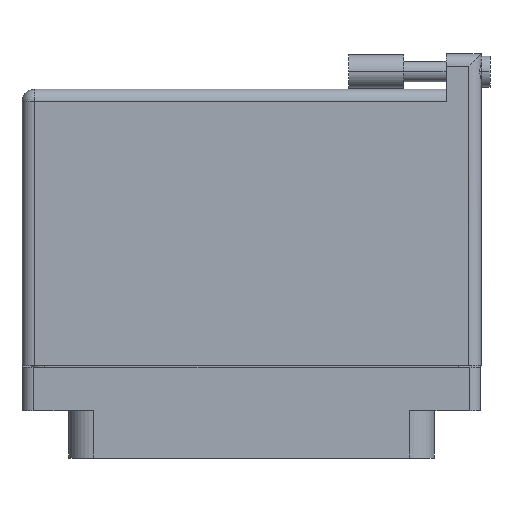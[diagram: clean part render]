
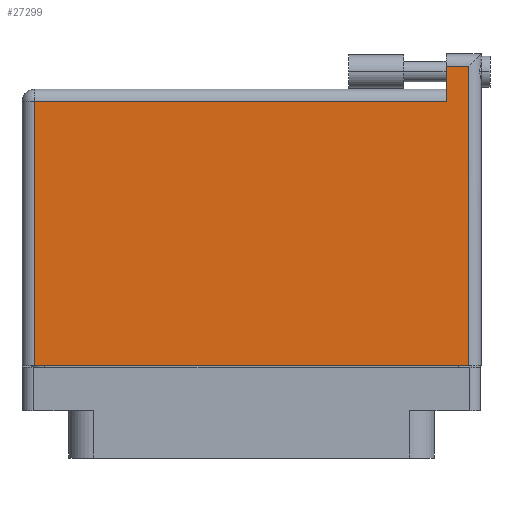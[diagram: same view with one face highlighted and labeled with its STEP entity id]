
A CAD part, front view. The second image highlights one B-rep face of the part: STEP entity #27299.
In plain terms, the highlighted face is planar.
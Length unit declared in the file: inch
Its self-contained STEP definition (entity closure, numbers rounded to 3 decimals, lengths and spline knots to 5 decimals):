
#318 = EDGE_LOOP ( 'NONE', ( #650, #1971, #25105, #33559, #22219, #26709 ) ) ;
#485 = DIRECTION ( 'NONE',  ( -1., 0., 0. ) ) ;
#650 = ORIENTED_EDGE ( 'NONE', *, *, #10344, .T. ) ;
#1971 = ORIENTED_EDGE ( 'NONE', *, *, #14185, .T. ) ;
#2944 = CARTESIAN_POINT ( 'NONE',  ( 1.23, 1.596, 0.4495 ) ) ;
#4171 = LINE ( 'NONE', #36304, #36687 ) ;
#6224 = CARTESIAN_POINT ( 'NONE',  ( -1.3, 1.396, 0.4495 ) ) ;
#7894 = CARTESIAN_POINT ( 'NONE',  ( -1.23, -0.1, 0.4495 ) ) ;
#9445 = VECTOR ( 'NONE', #18365, 39.37008 ) ;
#9795 = CARTESIAN_POINT ( 'NONE',  ( -1.3, 1.466, 0.4495 ) ) ;
#10344 = EDGE_CURVE ( 'NONE', #38540, #32235, #38788, .T. ) ;
#11542 = DIRECTION ( 'NONE',  ( 0., -1., 0. ) ) ;
#11992 = VECTOR ( 'NONE', #11542, 39.37008 ) ;
#13649 = LINE ( 'NONE', #29604, #9445 ) ;
#14185 = EDGE_CURVE ( 'NONE', #32235, #29164, #13649, .T. ) ;
#18365 = DIRECTION ( 'NONE',  ( 0., 1., 0. ) ) ;
#19514 = VERTEX_POINT ( 'NONE', #51599 ) ;
#22219 = ORIENTED_EDGE ( 'NONE', *, *, #42935, .T. ) ;
#25105 = ORIENTED_EDGE ( 'NONE', *, *, #32129, .T. ) ;
#25746 = PLANE ( 'NONE',  #43138 ) ;
#26006 = FACE_OUTER_BOUND ( 'NONE', #318, .T. ) ;
#26104 = LINE ( 'NONE', #6224, #44532 ) ;
#26105 = CARTESIAN_POINT ( 'NONE',  ( 1.23, -0.1, 0.4495 ) ) ;
#26254 = VECTOR ( 'NONE', #30962, 39.37008 ) ;
#26709 = ORIENTED_EDGE ( 'NONE', *, *, #37943, .T. ) ;
#27299 = ADVANCED_FACE ( 'NONE', ( #26006 ), #25746, .F. ) ;
#29164 = VERTEX_POINT ( 'NONE', #2944 ) ;
#29511 = DIRECTION ( 'NONE',  ( -1., 0., 0. ) ) ;
#29604 = CARTESIAN_POINT ( 'NONE',  ( 1.23, 1.666, 0.4495 ) ) ;
#30738 = CARTESIAN_POINT ( 'NONE',  ( 1.103, 1.666, 0.4495 ) ) ;
#30962 = DIRECTION ( 'NONE',  ( 1., 0., 0. ) ) ;
#32129 = EDGE_CURVE ( 'NONE', #29164, #34216, #4171, .T. ) ;
#32235 = VERTEX_POINT ( 'NONE', #26105 ) ;
#32478 = LINE ( 'NONE', #7894, #11992 ) ;
#32806 = EDGE_CURVE ( 'NONE', #34216, #33630, #34902, .T. ) ;
#32936 = CARTESIAN_POINT ( 'NONE',  ( -1.23, -0.1, 0.4495 ) ) ;
#33559 = ORIENTED_EDGE ( 'NONE', *, *, #32806, .T. ) ;
#33630 = VERTEX_POINT ( 'NONE', #35743 ) ;
#34216 = VERTEX_POINT ( 'NONE', #34673 ) ;
#34409 = DIRECTION ( 'NONE',  ( 0., -1., 0. ) ) ;
#34673 = CARTESIAN_POINT ( 'NONE',  ( 1.103, 1.596, 0.4495 ) ) ;
#34902 = LINE ( 'NONE', #30738, #40949 ) ;
#35743 = CARTESIAN_POINT ( 'NONE',  ( 1.103, 1.396, 0.4495 ) ) ;
#36304 = CARTESIAN_POINT ( 'NONE',  ( -1.3, 1.596, 0.4495 ) ) ;
#36687 = VECTOR ( 'NONE', #485, 39.37008 ) ;
#37943 = EDGE_CURVE ( 'NONE', #19514, #38540, #32478, .T. ) ;
#38540 = VERTEX_POINT ( 'NONE', #32936 ) ;
#38788 = LINE ( 'NONE', #39036, #26254 ) ;
#39036 = CARTESIAN_POINT ( 'NONE',  ( -1.3, -0.1, 0.4495 ) ) ;
#40949 = VECTOR ( 'NONE', #34409, 39.37008 ) ;
#41683 = DIRECTION ( 'NONE',  ( -1., 0., 0. ) ) ;
#42935 = EDGE_CURVE ( 'NONE', #33630, #19514, #26104, .T. ) ;
#43138 = AXIS2_PLACEMENT_3D ( 'NONE', #9795, #45093, #41683 ) ;
#44532 = VECTOR ( 'NONE', #29511, 39.37008 ) ;
#45093 = DIRECTION ( 'NONE',  ( 0., 0., -1. ) ) ;
#51599 = CARTESIAN_POINT ( 'NONE',  ( -1.23, 1.396, 0.4495 ) ) ;
